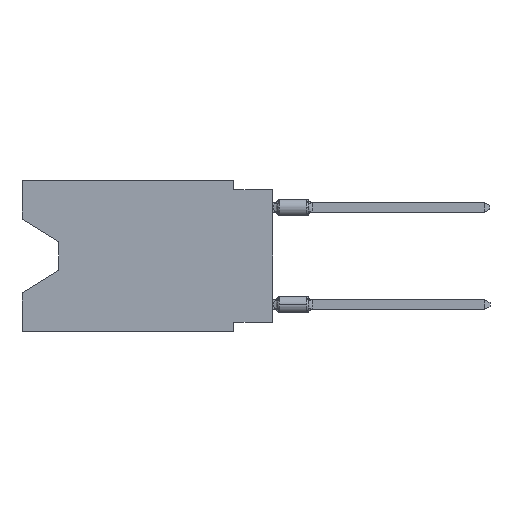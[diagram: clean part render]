
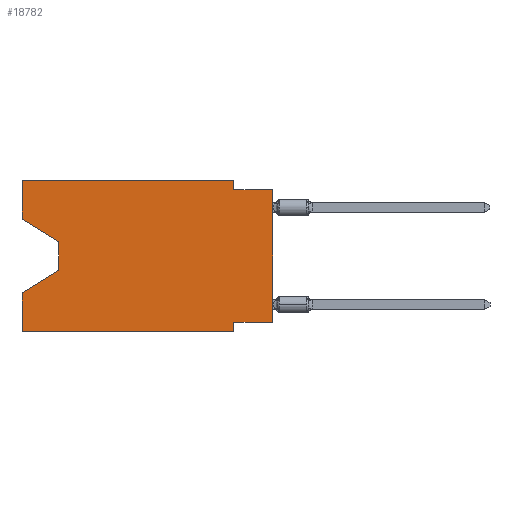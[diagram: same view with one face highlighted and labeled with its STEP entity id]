
A CAD part, left-side view. The second image highlights one B-rep face of the part: STEP entity #18782.
In plain terms, the highlighted planar face has unit normal (-1, 0, 0).
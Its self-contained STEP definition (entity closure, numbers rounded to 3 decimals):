
#95 = VECTOR ( 'NONE', #26539, 1000. ) ;
#295 = CARTESIAN_POINT ( 'NONE',  ( 0., 2.54, -9.906 ) ) ;
#366 = CARTESIAN_POINT ( 'NONE',  ( 0., 16.383, 0. ) ) ;
#448 = DIRECTION ( 'NONE',  ( 0., 0., -1. ) ) ;
#897 = VECTOR ( 'NONE', #20686, 1000. ) ;
#1504 = CARTESIAN_POINT ( 'NONE',  ( 0., 0., -0.635 ) ) ;
#1709 = VECTOR ( 'NONE', #21736, 1000. ) ;
#2075 = EDGE_CURVE ( 'NONE', #14734, #10469, #18332, .T. ) ;
#2230 = EDGE_CURVE ( 'NONE', #17187, #22286, #12676, .T. ) ;
#3141 = VECTOR ( 'NONE', #21946, 1000. ) ;
#3463 = LINE ( 'NONE', #27184, #897 ) ;
#4233 = LINE ( 'NONE', #12977, #1709 ) ;
#4509 = VERTEX_POINT ( 'NONE', #295 ) ;
#4614 = LINE ( 'NONE', #13361, #12042 ) ;
#4700 = CARTESIAN_POINT ( 'NONE',  ( 0., 16.383, 0. ) ) ;
#5303 = ORIENTED_EDGE ( 'NONE', *, *, #25872, .T. ) ;
#5424 = FACE_OUTER_BOUND ( 'NONE', #20114, .T. ) ;
#5663 = ORIENTED_EDGE ( 'NONE', *, *, #2075, .F. ) ;
#6279 = DIRECTION ( 'NONE',  ( 0., 0., 1. ) ) ;
#6282 = VERTEX_POINT ( 'NONE', #20646 ) ;
#7730 = DIRECTION ( 'NONE',  ( 0., 0., -1. ) ) ;
#7901 = CARTESIAN_POINT ( 'NONE',  ( 0., 16.383, -2.546 ) ) ;
#8541 = VECTOR ( 'NONE', #14697, 1000. ) ;
#8551 = VERTEX_POINT ( 'NONE', #13700 ) ;
#8879 = DIRECTION ( 'NONE',  ( 0., 0.855, -0.519 ) ) ;
#9029 = VECTOR ( 'NONE', #19193, 1000. ) ;
#9937 = VERTEX_POINT ( 'NONE', #7901 ) ;
#10172 = CARTESIAN_POINT ( 'NONE',  ( 0., 2.54, -9.271 ) ) ;
#10469 = VERTEX_POINT ( 'NONE', #12804 ) ;
#10603 = CARTESIAN_POINT ( 'NONE',  ( 0., 13.97, -5.893 ) ) ;
#10897 = LINE ( 'NONE', #11037, #23398 ) ;
#10910 = LINE ( 'NONE', #14782, #19124 ) ;
#11037 = CARTESIAN_POINT ( 'NONE',  ( 0., 13.97, -5.893 ) ) ;
#11363 = CARTESIAN_POINT ( 'NONE',  ( 0., 2.54, 0. ) ) ;
#11463 = CARTESIAN_POINT ( 'NONE',  ( 0., 16.383, 0. ) ) ;
#12042 = VECTOR ( 'NONE', #26322, 1000. ) ;
#12297 = CARTESIAN_POINT ( 'NONE',  ( 0., 0., 0. ) ) ;
#12676 = LINE ( 'NONE', #1504, #8541 ) ;
#12696 = LINE ( 'NONE', #12297, #9029 ) ;
#12804 = CARTESIAN_POINT ( 'NONE',  ( 0., 2.54, 0. ) ) ;
#12860 = ORIENTED_EDGE ( 'NONE', *, *, #2230, .F. ) ;
#12977 = CARTESIAN_POINT ( 'NONE',  ( 0., 16.383, -2.546 ) ) ;
#13361 = CARTESIAN_POINT ( 'NONE',  ( 0., 16.383, -9.906 ) ) ;
#13390 = ORIENTED_EDGE ( 'NONE', *, *, #25617, .F. ) ;
#13513 = EDGE_CURVE ( 'NONE', #10469, #17187, #16230, .T. ) ;
#13700 = CARTESIAN_POINT ( 'NONE',  ( 0., 0., -9.271 ) ) ;
#13830 = EDGE_CURVE ( 'NONE', #15442, #6282, #15595, .T. ) ;
#14164 = CARTESIAN_POINT ( 'NONE',  ( 0., 16.383, 0. ) ) ;
#14307 = CARTESIAN_POINT ( 'NONE',  ( 0., 13.97, -4.013 ) ) ;
#14517 = EDGE_CURVE ( 'NONE', #17201, #6282, #10897, .T. ) ;
#14697 = DIRECTION ( 'NONE',  ( 0., -1., 0. ) ) ;
#14734 = VERTEX_POINT ( 'NONE', #11463 ) ;
#14782 = CARTESIAN_POINT ( 'NONE',  ( 0., 0., -9.271 ) ) ;
#15197 = CARTESIAN_POINT ( 'NONE',  ( 0., 2.54, -0.635 ) ) ;
#15343 = LINE ( 'NONE', #19517, #3141 ) ;
#15442 = VERTEX_POINT ( 'NONE', #22310 ) ;
#15595 = LINE ( 'NONE', #366, #95 ) ;
#16230 = LINE ( 'NONE', #11363, #26718 ) ;
#16758 = EDGE_CURVE ( 'NONE', #15442, #4509, #4614, .T. ) ;
#17187 = VERTEX_POINT ( 'NONE', #15197 ) ;
#17201 = VERTEX_POINT ( 'NONE', #10603 ) ;
#17672 = ORIENTED_EDGE ( 'NONE', *, *, #25424, .T. ) ;
#18332 = LINE ( 'NONE', #20743, #23692 ) ;
#18782 = ADVANCED_FACE ( 'NONE', ( #5424 ), #22648, .F. ) ;
#19124 = VECTOR ( 'NONE', #26008, 1000. ) ;
#19193 = DIRECTION ( 'NONE',  ( 0., 0., 1. ) ) ;
#19517 = CARTESIAN_POINT ( 'NONE',  ( 0., 2.54, -9.906 ) ) ;
#19701 = CARTESIAN_POINT ( 'NONE',  ( 0., 0., -0.635 ) ) ;
#19905 = LINE ( 'NONE', #4700, #24724 ) ;
#20114 = EDGE_LOOP ( 'NONE', ( #22795, #17672, #27979, #21856, #25676, #26164, #13390, #5303, #12860, #27396, #5663, #26110 ) ) ;
#20332 = DIRECTION ( 'NONE',  ( 0., -1., 0. ) ) ;
#20646 = CARTESIAN_POINT ( 'NONE',  ( 0., 16.383, -7.36 ) ) ;
#20686 = DIRECTION ( 'NONE',  ( 0., 0., -1. ) ) ;
#20743 = CARTESIAN_POINT ( 'NONE',  ( 0., 16.383, 0. ) ) ;
#21736 = DIRECTION ( 'NONE',  ( 0., -0.855, -0.519 ) ) ;
#21856 = ORIENTED_EDGE ( 'NONE', *, *, #13830, .F. ) ;
#21946 = DIRECTION ( 'NONE',  ( 0., 0., -1. ) ) ;
#22286 = VERTEX_POINT ( 'NONE', #19701 ) ;
#22310 = CARTESIAN_POINT ( 'NONE',  ( 0., 16.383, -9.906 ) ) ;
#22512 = DIRECTION ( 'NONE',  ( 1., 0., 0. ) ) ;
#22648 = PLANE ( 'NONE',  #27323 ) ;
#22795 = ORIENTED_EDGE ( 'NONE', *, *, #26000, .T. ) ;
#23398 = VECTOR ( 'NONE', #8879, 1000. ) ;
#23692 = VECTOR ( 'NONE', #20332, 1000. ) ;
#24013 = EDGE_CURVE ( 'NONE', #24272, #4509, #15343, .T. ) ;
#24272 = VERTEX_POINT ( 'NONE', #10172 ) ;
#24401 = EDGE_CURVE ( 'NONE', #9937, #14734, #19905, .T. ) ;
#24724 = VECTOR ( 'NONE', #6279, 1000. ) ;
#25424 = EDGE_CURVE ( 'NONE', #27655, #17201, #3463, .T. ) ;
#25617 = EDGE_CURVE ( 'NONE', #8551, #24272, #10910, .T. ) ;
#25676 = ORIENTED_EDGE ( 'NONE', *, *, #16758, .T. ) ;
#25872 = EDGE_CURVE ( 'NONE', #8551, #22286, #12696, .T. ) ;
#26000 = EDGE_CURVE ( 'NONE', #9937, #27655, #4233, .T. ) ;
#26008 = DIRECTION ( 'NONE',  ( 0., 1., 0. ) ) ;
#26110 = ORIENTED_EDGE ( 'NONE', *, *, #24401, .F. ) ;
#26164 = ORIENTED_EDGE ( 'NONE', *, *, #24013, .F. ) ;
#26322 = DIRECTION ( 'NONE',  ( 0., -1., 0. ) ) ;
#26539 = DIRECTION ( 'NONE',  ( 0., 0., 1. ) ) ;
#26718 = VECTOR ( 'NONE', #448, 1000. ) ;
#27184 = CARTESIAN_POINT ( 'NONE',  ( 0., 13.97, -4.013 ) ) ;
#27323 = AXIS2_PLACEMENT_3D ( 'NONE', #14164, #22512, #7730 ) ;
#27396 = ORIENTED_EDGE ( 'NONE', *, *, #13513, .F. ) ;
#27655 = VERTEX_POINT ( 'NONE', #14307 ) ;
#27979 = ORIENTED_EDGE ( 'NONE', *, *, #14517, .T. ) ;
